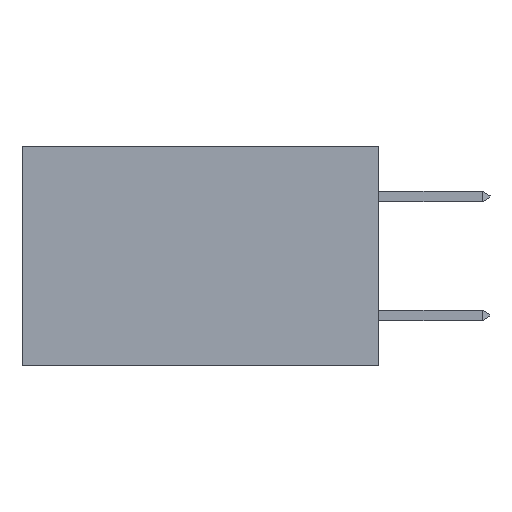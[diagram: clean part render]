
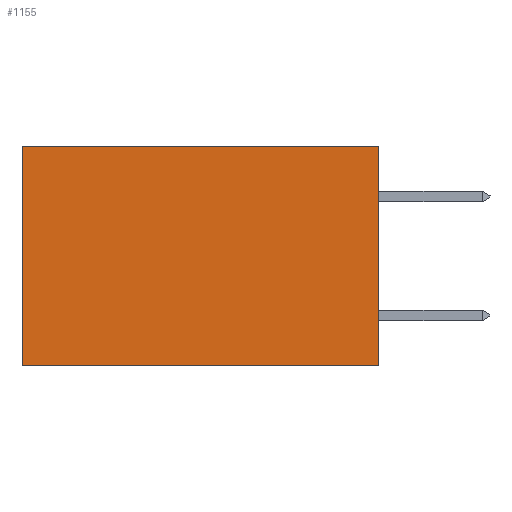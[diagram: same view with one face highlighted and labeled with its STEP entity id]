
A CAD part, left-side view. The second image highlights one B-rep face of the part: STEP entity #1155.
In plain terms, the highlighted planar face has unit normal (-1, 0, 0).
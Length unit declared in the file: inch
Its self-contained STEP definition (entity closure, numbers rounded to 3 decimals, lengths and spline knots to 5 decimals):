
#617 = VERTEX_POINT ( 'NONE', #4542 ) ;
#774 = DIRECTION ( 'NONE',  ( 0., 1., 0. ) ) ;
#1155 = ADVANCED_FACE ( 'NONE', ( #5192 ), #15679, .F. ) ;
#1435 = EDGE_CURVE ( 'NONE', #617, #2181, #10979, .T. ) ;
#1718 = ORIENTED_EDGE ( 'NONE', *, *, #9175, .T. ) ;
#1766 = VECTOR ( 'NONE', #774, 39.37008 ) ;
#1978 = CARTESIAN_POINT ( 'NONE',  ( 0.2615, 0., -0.37 ) ) ;
#2181 = VERTEX_POINT ( 'NONE', #10046 ) ;
#2523 = DIRECTION ( 'NONE',  ( 0., 0., -1. ) ) ;
#3646 = EDGE_LOOP ( 'NONE', ( #1718, #4166, #16074, #14165 ) ) ;
#3847 = LINE ( 'NONE', #6617, #7956 ) ;
#4166 = ORIENTED_EDGE ( 'NONE', *, *, #1435, .F. ) ;
#4277 = EDGE_CURVE ( 'NONE', #9117, #617, #5859, .T. ) ;
#4542 = CARTESIAN_POINT ( 'NONE',  ( 0.2615, 0., -0.37 ) ) ;
#4947 = DIRECTION ( 'NONE',  ( 1., 0., 0. ) ) ;
#5192 = FACE_OUTER_BOUND ( 'NONE', #3646, .T. ) ;
#5792 = VERTEX_POINT ( 'NONE', #7269 ) ;
#5859 = LINE ( 'NONE', #1978, #7629 ) ;
#6617 = CARTESIAN_POINT ( 'NONE',  ( 0.2615, 0.6, -0.37 ) ) ;
#6687 = DIRECTION ( 'NONE',  ( 0., 0., -1. ) ) ;
#7243 = DIRECTION ( 'NONE',  ( 0., 0., -1. ) ) ;
#7269 = CARTESIAN_POINT ( 'NONE',  ( 0.2615, 0.6, 0. ) ) ;
#7629 = VECTOR ( 'NONE', #7243, 39.37008 ) ;
#7956 = VECTOR ( 'NONE', #6687, 39.37008 ) ;
#8592 = LINE ( 'NONE', #14393, #10370 ) ;
#9117 = VERTEX_POINT ( 'NONE', #16945 ) ;
#9175 = EDGE_CURVE ( 'NONE', #5792, #2181, #3847, .T. ) ;
#9848 = CARTESIAN_POINT ( 'NONE',  ( 0.2615, 0., -0.37 ) ) ;
#10046 = CARTESIAN_POINT ( 'NONE',  ( 0.2615, 0.6, -0.37 ) ) ;
#10370 = VECTOR ( 'NONE', #11524, 39.37008 ) ;
#10979 = LINE ( 'NONE', #9848, #1766 ) ;
#11524 = DIRECTION ( 'NONE',  ( 0., 1., 0. ) ) ;
#12327 = EDGE_CURVE ( 'NONE', #9117, #5792, #8592, .T. ) ;
#12938 = AXIS2_PLACEMENT_3D ( 'NONE', #14203, #4947, #2523 ) ;
#14165 = ORIENTED_EDGE ( 'NONE', *, *, #12327, .T. ) ;
#14203 = CARTESIAN_POINT ( 'NONE',  ( 0.2615, 0., -0.37 ) ) ;
#14393 = CARTESIAN_POINT ( 'NONE',  ( 0.2615, 0., 0. ) ) ;
#15679 = PLANE ( 'NONE',  #12938 ) ;
#16074 = ORIENTED_EDGE ( 'NONE', *, *, #4277, .F. ) ;
#16945 = CARTESIAN_POINT ( 'NONE',  ( 0.2615, 0., 0. ) ) ;
